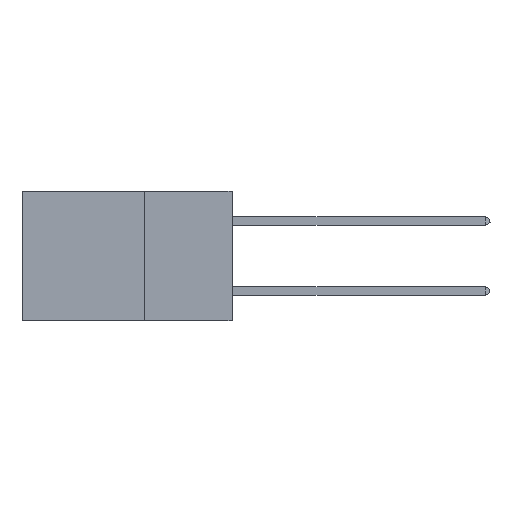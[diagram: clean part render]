
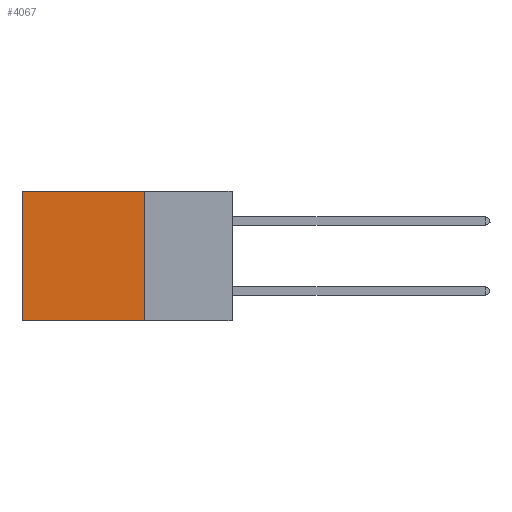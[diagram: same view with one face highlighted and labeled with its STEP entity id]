
A CAD part, left-side view. The second image highlights one B-rep face of the part: STEP entity #4067.
In plain terms, the highlighted planar face has unit normal (-1, 0, 0).
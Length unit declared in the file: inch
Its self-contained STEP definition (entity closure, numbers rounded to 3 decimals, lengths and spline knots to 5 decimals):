
#287 = ORIENTED_EDGE ( 'NONE', *, *, #26263, .F. ) ;
#786 = EDGE_CURVE ( 'NONE', #5840, #32979, #30293, .T. ) ;
#3932 = LINE ( 'NONE', #35425, #12762 ) ;
#4067 = ADVANCED_FACE ( 'NONE', ( #18138 ), #25445, .F. ) ;
#4991 = CARTESIAN_POINT ( 'NONE',  ( 0.2875, 0.25, 0. ) ) ;
#5427 = EDGE_LOOP ( 'NONE', ( #28848, #7885, #287, #11399 ) ) ;
#5840 = VERTEX_POINT ( 'NONE', #25400 ) ;
#6138 = CARTESIAN_POINT ( 'NONE',  ( 0.2875, 0.25, 0. ) ) ;
#7691 = VECTOR ( 'NONE', #20175, 39.37008 ) ;
#7885 = ORIENTED_EDGE ( 'NONE', *, *, #786, .F. ) ;
#9610 = DIRECTION ( 'NONE',  ( 0., 0., -1. ) ) ;
#11399 = ORIENTED_EDGE ( 'NONE', *, *, #21629, .T. ) ;
#12762 = VECTOR ( 'NONE', #9610, 39.37008 ) ;
#13725 = CARTESIAN_POINT ( 'NONE',  ( 0.2875, 0.25, -0.37 ) ) ;
#15008 = EDGE_CURVE ( 'NONE', #37813, #32979, #28165, .T. ) ;
#15118 = DIRECTION ( 'NONE',  ( 1., 0., 0. ) ) ;
#15759 = DIRECTION ( 'NONE',  ( 0., 0., -1. ) ) ;
#18017 = CARTESIAN_POINT ( 'NONE',  ( 0.2875, 0.6, -0.37 ) ) ;
#18049 = CARTESIAN_POINT ( 'NONE',  ( 0.2875, 0.6, 0. ) ) ;
#18138 = FACE_OUTER_BOUND ( 'NONE', #5427, .T. ) ;
#20175 = DIRECTION ( 'NONE',  ( 0., 1., 0. ) ) ;
#21629 = EDGE_CURVE ( 'NONE', #40137, #37813, #26045, .T. ) ;
#23920 = AXIS2_PLACEMENT_3D ( 'NONE', #4991, #15118, #15759 ) ;
#24310 = VECTOR ( 'NONE', #32490, 39.37008 ) ;
#25129 = DIRECTION ( 'NONE',  ( 0., 0., -1. ) ) ;
#25400 = CARTESIAN_POINT ( 'NONE',  ( 0.2875, 0.25, -0.37 ) ) ;
#25445 = PLANE ( 'NONE',  #23920 ) ;
#26045 = LINE ( 'NONE', #41963, #24310 ) ;
#26263 = EDGE_CURVE ( 'NONE', #40137, #5840, #3932, .T. ) ;
#28165 = LINE ( 'NONE', #18049, #35586 ) ;
#28848 = ORIENTED_EDGE ( 'NONE', *, *, #15008, .T. ) ;
#30293 = LINE ( 'NONE', #13725, #7691 ) ;
#32490 = DIRECTION ( 'NONE',  ( 0., 1., 0. ) ) ;
#32979 = VERTEX_POINT ( 'NONE', #18017 ) ;
#35425 = CARTESIAN_POINT ( 'NONE',  ( 0.2875, 0.25, 0. ) ) ;
#35506 = CARTESIAN_POINT ( 'NONE',  ( 0.2875, 0.6, 0. ) ) ;
#35586 = VECTOR ( 'NONE', #25129, 39.37008 ) ;
#37813 = VERTEX_POINT ( 'NONE', #35506 ) ;
#40137 = VERTEX_POINT ( 'NONE', #6138 ) ;
#41963 = CARTESIAN_POINT ( 'NONE',  ( 0.2875, 0.25, 0. ) ) ;
